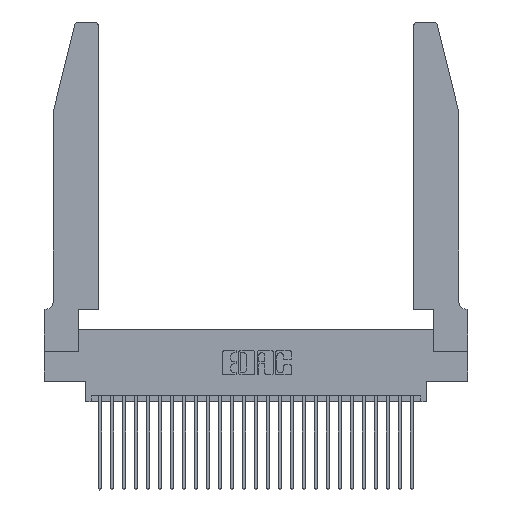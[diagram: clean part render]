
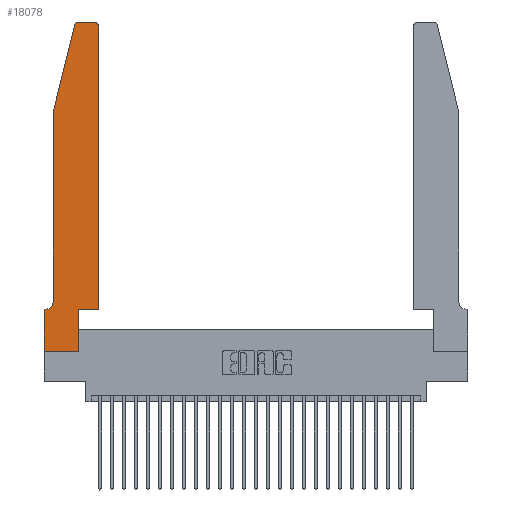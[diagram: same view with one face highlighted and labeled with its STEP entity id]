
A CAD part, top view. The second image highlights one B-rep face of the part: STEP entity #18078.
In plain terms, the highlighted planar face has unit normal (0, 0, 1).
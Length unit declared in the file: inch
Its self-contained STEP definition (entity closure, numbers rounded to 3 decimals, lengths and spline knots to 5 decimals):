
#605 = VECTOR ( 'NONE', #3487, 39.37008 ) ;
#1657 = VECTOR ( 'NONE', #2808, 39.37008 ) ;
#1778 = ORIENTED_EDGE ( 'NONE', *, *, #7828, .T. ) ;
#1913 = VERTEX_POINT ( 'NONE', #20399 ) ;
#2163 = VECTOR ( 'NONE', #16652, 39.37008 ) ;
#2301 = DIRECTION ( 'NONE',  ( 0., 0., 1. ) ) ;
#2808 = DIRECTION ( 'NONE',  ( -1., 0., 0. ) ) ;
#2898 = EDGE_CURVE ( 'NONE', #6876, #21393, #5520, .T. ) ;
#3244 = FACE_OUTER_BOUND ( 'NONE', #25980, .T. ) ;
#3487 = DIRECTION ( 'NONE',  ( 0., 1., 0. ) ) ;
#3730 = DIRECTION ( 'NONE',  ( -1., 0., 0. ) ) ;
#3795 = EDGE_CURVE ( 'NONE', #14504, #6876, #23148, .T. ) ;
#4208 = LINE ( 'NONE', #12378, #2163 ) ;
#4559 = LINE ( 'NONE', #24812, #12736 ) ;
#4637 = EDGE_CURVE ( 'NONE', #6282, #14504, #25418, .T. ) ;
#4781 = VERTEX_POINT ( 'NONE', #19153 ) ;
#5021 = CIRCLE ( 'NONE', #27115, 0.03 ) ;
#5405 = EDGE_CURVE ( 'NONE', #10978, #4781, #23674, .T. ) ;
#5520 = LINE ( 'NONE', #24146, #15718 ) ;
#5702 = EDGE_CURVE ( 'NONE', #4781, #7153, #6672, .T. ) ;
#5792 = CARTESIAN_POINT ( 'NONE',  ( 0.0755, 2., 0.37 ) ) ;
#6282 = VERTEX_POINT ( 'NONE', #26143 ) ;
#6415 = CARTESIAN_POINT ( 'NONE',  ( 0.4205, 2.72, 0.37 ) ) ;
#6672 = CIRCLE ( 'NONE', #22219, 0.07 ) ;
#6876 = VERTEX_POINT ( 'NONE', #17664 ) ;
#7153 = VERTEX_POINT ( 'NONE', #23645 ) ;
#7338 = ORIENTED_EDGE ( 'NONE', *, *, #4637, .T. ) ;
#7828 = EDGE_CURVE ( 'NONE', #18115, #14868, #27239, .T. ) ;
#7919 = VERTEX_POINT ( 'NONE', #12971 ) ;
#8124 = ORIENTED_EDGE ( 'NONE', *, *, #13395, .T. ) ;
#8148 = DIRECTION ( 'NONE',  ( 0., -1., 0. ) ) ;
#9418 = CARTESIAN_POINT ( 'NONE',  ( 0.4505, 2.72, 0.37 ) ) ;
#10114 = CARTESIAN_POINT ( 'NONE',  ( 0.0055, 0.42, 0.37 ) ) ;
#10145 = DIRECTION ( 'NONE',  ( 0., 0., 1. ) ) ;
#10357 = EDGE_CURVE ( 'NONE', #21393, #1913, #5021, .T. ) ;
#10433 = VECTOR ( 'NONE', #8148, 39.37008 ) ;
#10978 = VERTEX_POINT ( 'NONE', #5792 ) ;
#11026 = CARTESIAN_POINT ( 'NONE',  ( 0.2865, 0., 0.37 ) ) ;
#12299 = DIRECTION ( 'NONE',  ( 0., 0., -1. ) ) ;
#12378 = CARTESIAN_POINT ( 'NONE',  ( 0., 0., 0.37 ) ) ;
#12651 = CARTESIAN_POINT ( 'NONE',  ( 0., 0., 0.37 ) ) ;
#12692 = ORIENTED_EDGE ( 'NONE', *, *, #10357, .T. ) ;
#12736 = VECTOR ( 'NONE', #26803, 39.37008 ) ;
#12971 = CARTESIAN_POINT ( 'NONE',  ( 0., 0., 0.37 ) ) ;
#13395 = EDGE_CURVE ( 'NONE', #7153, #26816, #14584, .T. ) ;
#13417 = ORIENTED_EDGE ( 'NONE', *, *, #5702, .T. ) ;
#13705 = CARTESIAN_POINT ( 'NONE',  ( 0.284, 2.75, 0.37 ) ) ;
#13833 = AXIS2_PLACEMENT_3D ( 'NONE', #6415, #2301, #17505 ) ;
#13984 = CARTESIAN_POINT ( 'NONE',  ( 0.4505, 0.35, 0.37 ) ) ;
#14078 = ORIENTED_EDGE ( 'NONE', *, *, #17553, .T. ) ;
#14504 = VERTEX_POINT ( 'NONE', #9418 ) ;
#14584 = LINE ( 'NONE', #23635, #1657 ) ;
#14868 = VERTEX_POINT ( 'NONE', #15694 ) ;
#15197 = EDGE_CURVE ( 'NONE', #14868, #6282, #17182, .T. ) ;
#15694 = CARTESIAN_POINT ( 'NONE',  ( 0.2865, 0.35, 0.37 ) ) ;
#15718 = VECTOR ( 'NONE', #16083, 39.37008 ) ;
#16083 = DIRECTION ( 'NONE',  ( -1., 0., 0. ) ) ;
#16532 = CARTESIAN_POINT ( 'NONE',  ( 0.4505, 0.35, 0.37 ) ) ;
#16652 = DIRECTION ( 'NONE',  ( 0., -1., 0. ) ) ;
#17012 = DIRECTION ( 'NONE',  ( 1., 0., 0. ) ) ;
#17182 = LINE ( 'NONE', #13984, #17495 ) ;
#17288 = DIRECTION ( 'NONE',  ( 1., 0., 0. ) ) ;
#17367 = CARTESIAN_POINT ( 'NONE',  ( 0., 0.35, 0.37 ) ) ;
#17495 = VECTOR ( 'NONE', #17288, 39.37008 ) ;
#17505 = DIRECTION ( 'NONE',  ( 1., 0., 0. ) ) ;
#17553 = EDGE_CURVE ( 'NONE', #7919, #18115, #24569, .T. ) ;
#17664 = CARTESIAN_POINT ( 'NONE',  ( 0.4205, 2.75, 0.37 ) ) ;
#18078 = ADVANCED_FACE ( 'NONE', ( #3244 ), #21722, .T. ) ;
#18115 = VERTEX_POINT ( 'NONE', #11026 ) ;
#19040 = EDGE_CURVE ( 'NONE', #26816, #7919, #4208, .T. ) ;
#19153 = CARTESIAN_POINT ( 'NONE',  ( 0.0755, 0.42, 0.37 ) ) ;
#19441 = DIRECTION ( 'NONE',  ( 0., 0., 1. ) ) ;
#19522 = ORIENTED_EDGE ( 'NONE', *, *, #15197, .T. ) ;
#19695 = CARTESIAN_POINT ( 'NONE',  ( 0., 0.35, 0.37 ) ) ;
#19901 = ORIENTED_EDGE ( 'NONE', *, *, #19040, .T. ) ;
#20160 = VECTOR ( 'NONE', #17012, 39.37008 ) ;
#20399 = CARTESIAN_POINT ( 'NONE',  ( 0.25487, 2.72718, 0.37 ) ) ;
#20966 = CARTESIAN_POINT ( 'NONE',  ( 0.284, 2.72, 0.37 ) ) ;
#21210 = CARTESIAN_POINT ( 'NONE',  ( 0.0755, 2., 0.37 ) ) ;
#21393 = VERTEX_POINT ( 'NONE', #13705 ) ;
#21566 = ORIENTED_EDGE ( 'NONE', *, *, #3795, .T. ) ;
#21651 = CARTESIAN_POINT ( 'NONE',  ( 0.2865, 0.35, 0.37 ) ) ;
#21722 = PLANE ( 'NONE',  #26334 ) ;
#21992 = ORIENTED_EDGE ( 'NONE', *, *, #5405, .T. ) ;
#22219 = AXIS2_PLACEMENT_3D ( 'NONE', #10114, #12299, #3730 ) ;
#22845 = VECTOR ( 'NONE', #24028, 39.37008 ) ;
#23148 = CIRCLE ( 'NONE', #13833, 0.03 ) ;
#23542 = DIRECTION ( 'NONE',  ( 1., 0., 0. ) ) ;
#23635 = CARTESIAN_POINT ( 'NONE',  ( 0.0755, 0.35, 0.37 ) ) ;
#23645 = CARTESIAN_POINT ( 'NONE',  ( 0.0055, 0.35, 0.37 ) ) ;
#23674 = LINE ( 'NONE', #21210, #10433 ) ;
#24028 = DIRECTION ( 'NONE',  ( 0., 1., 0. ) ) ;
#24146 = CARTESIAN_POINT ( 'NONE',  ( 0.2605, 2.75, 0.37 ) ) ;
#24569 = LINE ( 'NONE', #12651, #20160 ) ;
#24812 = CARTESIAN_POINT ( 'NONE',  ( 0.0755, 2., 0.37 ) ) ;
#25106 = ORIENTED_EDGE ( 'NONE', *, *, #26368, .T. ) ;
#25418 = LINE ( 'NONE', #16532, #605 ) ;
#25980 = EDGE_LOOP ( 'NONE', ( #28131, #12692, #25106, #21992, #13417, #8124, #19901, #14078, #1778, #19522, #7338, #21566 ) ) ;
#26143 = CARTESIAN_POINT ( 'NONE',  ( 0.4505, 0.35, 0.37 ) ) ;
#26334 = AXIS2_PLACEMENT_3D ( 'NONE', #17367, #19441, #23542 ) ;
#26368 = EDGE_CURVE ( 'NONE', #1913, #10978, #4559, .T. ) ;
#26803 = DIRECTION ( 'NONE',  ( -0.239, -0.971, 0. ) ) ;
#26816 = VERTEX_POINT ( 'NONE', #19695 ) ;
#27115 = AXIS2_PLACEMENT_3D ( 'NONE', #20966, #10145, #27501 ) ;
#27239 = LINE ( 'NONE', #21651, #22845 ) ;
#27501 = DIRECTION ( 'NONE',  ( 1., 0., 0. ) ) ;
#28131 = ORIENTED_EDGE ( 'NONE', *, *, #2898, .T. ) ;
